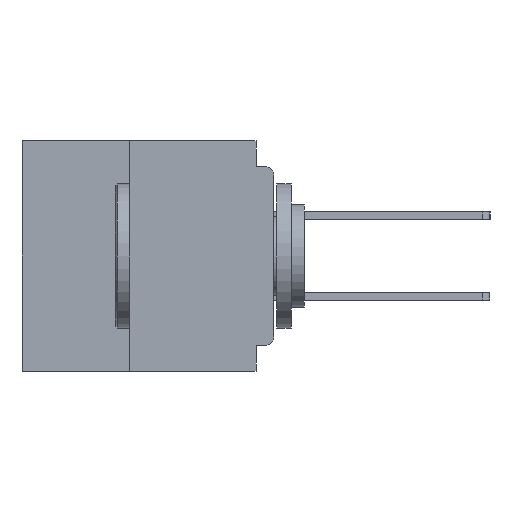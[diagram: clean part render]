
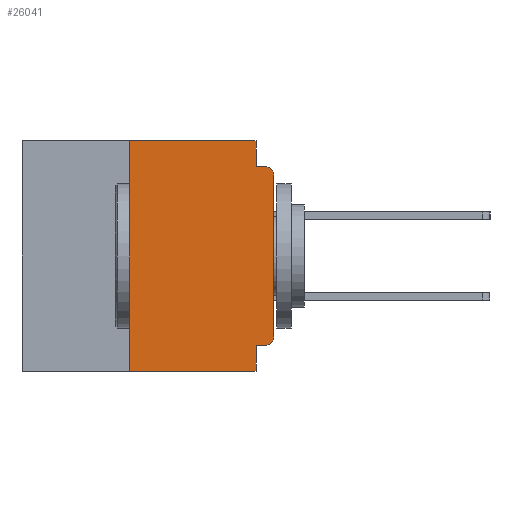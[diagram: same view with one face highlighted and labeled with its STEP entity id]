
A CAD part, left-side view. The second image highlights one B-rep face of the part: STEP entity #26041.
In plain terms, the highlighted planar face has unit normal (-1, 0, 0).
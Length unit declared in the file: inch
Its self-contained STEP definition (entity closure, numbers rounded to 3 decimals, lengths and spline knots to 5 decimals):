
#497 = LINE ( 'NONE', #23035, #25488 ) ;
#1819 = VERTEX_POINT ( 'NONE', #35691 ) ;
#1941 = AXIS2_PLACEMENT_3D ( 'NONE', #32828, #13383, #36100 ) ;
#2399 = LINE ( 'NONE', #34256, #36003 ) ;
#2537 = CARTESIAN_POINT ( 'NONE',  ( 0., 0., -0.06 ) ) ;
#2633 = ORIENTED_EDGE ( 'NONE', *, *, #24236, .F. ) ;
#2710 = CARTESIAN_POINT ( 'NONE',  ( 0., 0.25, -0.4 ) ) ;
#2774 = ORIENTED_EDGE ( 'NONE', *, *, #27002, .T. ) ;
#2939 = ORIENTED_EDGE ( 'NONE', *, *, #14278, .F. ) ;
#3047 = VECTOR ( 'NONE', #36103, 39.37008 ) ;
#3945 = VERTEX_POINT ( 'NONE', #36275 ) ;
#3985 = EDGE_CURVE ( 'NONE', #16854, #9154, #497, .T. ) ;
#5136 = LINE ( 'NONE', #13386, #3047 ) ;
#5219 = ORIENTED_EDGE ( 'NONE', *, *, #34928, .T. ) ;
#5273 = ORIENTED_EDGE ( 'NONE', *, *, #3985, .F. ) ;
#5395 = VERTEX_POINT ( 'NONE', #10166 ) ;
#5410 = DIRECTION ( 'NONE',  ( 0., -1., 0. ) ) ;
#5980 = AXIS2_PLACEMENT_3D ( 'NONE', #21366, #8418, #31135 ) ;
#8418 = DIRECTION ( 'NONE',  ( 1., 0., 0. ) ) ;
#8895 = DIRECTION ( 'NONE',  ( 0., 1., 0. ) ) ;
#9154 = VERTEX_POINT ( 'NONE', #37300 ) ;
#9898 = VECTOR ( 'NONE', #28033, 39.37008 ) ;
#9975 = VERTEX_POINT ( 'NONE', #28285 ) ;
#10166 = CARTESIAN_POINT ( 'NONE',  ( 0., 0.25, -0.4 ) ) ;
#10698 = DIRECTION ( 'NONE',  ( 0., -1., 0. ) ) ;
#12377 = VERTEX_POINT ( 'NONE', #31842 ) ;
#12575 = DIRECTION ( 'NONE',  ( 0., 0., 1. ) ) ;
#13092 = CARTESIAN_POINT ( 'NONE',  ( 0., 0.031, -0.4 ) ) ;
#13383 = DIRECTION ( 'NONE',  ( -1., 0., 0. ) ) ;
#13386 = CARTESIAN_POINT ( 'NONE',  ( 0., 0.031, -0.4 ) ) ;
#13663 = LINE ( 'NONE', #34877, #38556 ) ;
#13705 = CARTESIAN_POINT ( 'NONE',  ( 0., 0.437, -0.4 ) ) ;
#14278 = EDGE_CURVE ( 'NONE', #35892, #3945, #19787, .T. ) ;
#14923 = VECTOR ( 'NONE', #12575, 39.37008 ) ;
#15247 = DIRECTION ( 'NONE',  ( -1., 0., 0. ) ) ;
#16854 = VERTEX_POINT ( 'NONE', #24780 ) ;
#17404 = LINE ( 'NONE', #13705, #41283 ) ;
#18328 = EDGE_CURVE ( 'NONE', #5395, #35892, #25590, .T. ) ;
#18375 = CARTESIAN_POINT ( 'NONE',  ( 0., 0.437, 0. ) ) ;
#19787 = LINE ( 'NONE', #18375, #33978 ) ;
#21366 = CARTESIAN_POINT ( 'NONE',  ( 0., 0.437, 0. ) ) ;
#22188 = CIRCLE ( 'NONE', #1941, 0.015 ) ;
#22366 = ORIENTED_EDGE ( 'NONE', *, *, #18328, .F. ) ;
#23035 = CARTESIAN_POINT ( 'NONE',  ( 0., 0., -0.045 ) ) ;
#23296 = CARTESIAN_POINT ( 'NONE',  ( 0., 0.25, 0. ) ) ;
#23781 = DIRECTION ( 'NONE',  ( 0., -1., 0. ) ) ;
#24236 = EDGE_CURVE ( 'NONE', #3945, #16854, #2399, .T. ) ;
#24626 = DIRECTION ( 'NONE',  ( 0., 0., -1. ) ) ;
#24780 = CARTESIAN_POINT ( 'NONE',  ( 0., 0.031, -0.045 ) ) ;
#24787 = CARTESIAN_POINT ( 'NONE',  ( 0., 0., 0. ) ) ;
#25488 = VECTOR ( 'NONE', #23781, 39.37008 ) ;
#25590 = LINE ( 'NONE', #2710, #14923 ) ;
#26041 = ADVANCED_FACE ( 'NONE', ( #28230 ), #31000, .F. ) ;
#26190 = LINE ( 'NONE', #24787, #9898 ) ;
#26902 = ORIENTED_EDGE ( 'NONE', *, *, #28559, .F. ) ;
#27002 = EDGE_CURVE ( 'NONE', #5395, #27491, #17404, .T. ) ;
#27491 = VERTEX_POINT ( 'NONE', #13092 ) ;
#28033 = DIRECTION ( 'NONE',  ( 0., 0., 1. ) ) ;
#28230 = FACE_OUTER_BOUND ( 'NONE', #28889, .T. ) ;
#28285 = CARTESIAN_POINT ( 'NONE',  ( 0., 0.031, -0.355 ) ) ;
#28559 = EDGE_CURVE ( 'NONE', #12377, #9975, #13663, .T. ) ;
#28889 = EDGE_LOOP ( 'NONE', ( #39347, #30716, #5273, #2633, #2939, #22366, #2774, #40110, #26902, #5219 ) ) ;
#29126 = VERTEX_POINT ( 'NONE', #2537 ) ;
#29904 = EDGE_CURVE ( 'NONE', #29126, #9154, #22188, .T. ) ;
#30260 = CIRCLE ( 'NONE', #36973, 0.015 ) ;
#30716 = ORIENTED_EDGE ( 'NONE', *, *, #29904, .T. ) ;
#31000 = PLANE ( 'NONE',  #5980 ) ;
#31135 = DIRECTION ( 'NONE',  ( 0., 0., -1. ) ) ;
#31842 = CARTESIAN_POINT ( 'NONE',  ( 0., 0.015, -0.355 ) ) ;
#32828 = CARTESIAN_POINT ( 'NONE',  ( 0., 0.015, -0.06 ) ) ;
#33978 = VECTOR ( 'NONE', #5410, 39.37008 ) ;
#34256 = CARTESIAN_POINT ( 'NONE',  ( 0., 0.031, 0. ) ) ;
#34682 = CARTESIAN_POINT ( 'NONE',  ( 0., 0.015, -0.34 ) ) ;
#34877 = CARTESIAN_POINT ( 'NONE',  ( 0., 0., -0.355 ) ) ;
#34928 = EDGE_CURVE ( 'NONE', #12377, #1819, #30260, .T. ) ;
#35002 = EDGE_CURVE ( 'NONE', #1819, #29126, #26190, .T. ) ;
#35691 = CARTESIAN_POINT ( 'NONE',  ( 0., 0., -0.34 ) ) ;
#35892 = VERTEX_POINT ( 'NONE', #23296 ) ;
#36003 = VECTOR ( 'NONE', #24626, 39.37008 ) ;
#36100 = DIRECTION ( 'NONE',  ( 0., 0., -1. ) ) ;
#36103 = DIRECTION ( 'NONE',  ( 0., 0., -1. ) ) ;
#36275 = CARTESIAN_POINT ( 'NONE',  ( 0., 0.031, 0. ) ) ;
#36973 = AXIS2_PLACEMENT_3D ( 'NONE', #34682, #15247, #37957 ) ;
#37136 = EDGE_CURVE ( 'NONE', #9975, #27491, #5136, .T. ) ;
#37300 = CARTESIAN_POINT ( 'NONE',  ( 0., 0.015, -0.045 ) ) ;
#37957 = DIRECTION ( 'NONE',  ( 0., 0., -1. ) ) ;
#38556 = VECTOR ( 'NONE', #8895, 39.37008 ) ;
#39347 = ORIENTED_EDGE ( 'NONE', *, *, #35002, .T. ) ;
#40110 = ORIENTED_EDGE ( 'NONE', *, *, #37136, .F. ) ;
#41283 = VECTOR ( 'NONE', #10698, 39.37008 ) ;
